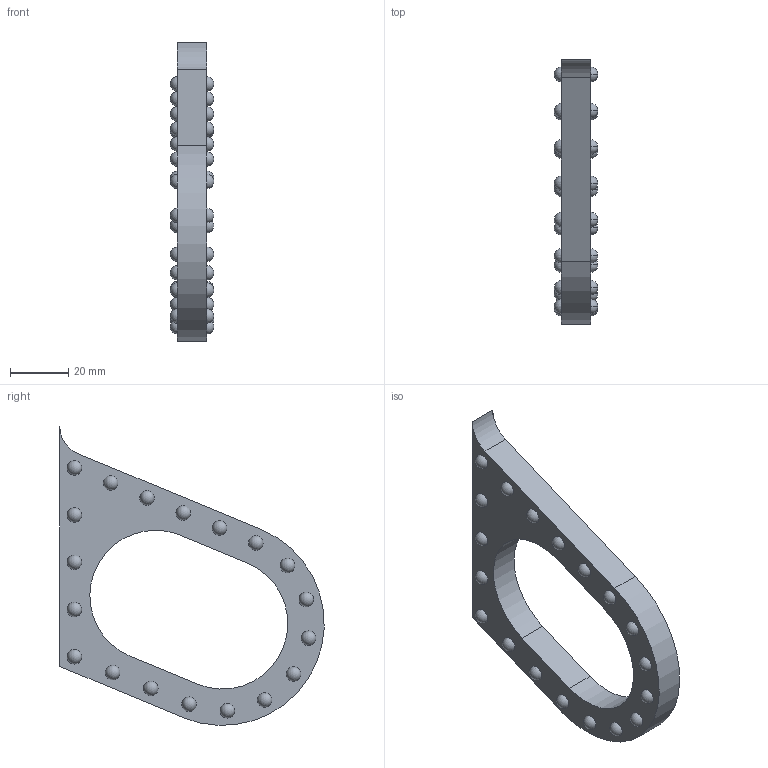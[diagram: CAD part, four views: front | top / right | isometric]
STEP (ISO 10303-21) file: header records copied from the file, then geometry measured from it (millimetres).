
FILE_DESCRIPTION (( 'STEP AP214' ), '1' );
FILE_NAME ('Grip_Middle.step', '2013-11-06T14:31:01', ( 'elpi' ), ( '' ), 'SwSTEP 2.0', 'SolidWorks 2013', '' );
FILE_SCHEMA (( 'AUTOMOTIVE_DESIGN' ));
Length unit declared in the file: millimetre
Products named in the file (1): Grip_Middle
Bounding box: 14.98 x 90.86 x 102.69 mm (x, y, z)
Volume: 35762.4 mm3; surface area: 12748.7 mm2
Topology: 1 solids, 1 shells, 69 faces, 277 edges, 172 vertices
Faces by surface type: sphere 57, plane 7, cylinder 5
Entity records: 1846 total; most frequent: DIRECTION 370, CARTESIAN_POINT 291, ORIENTED_EDGE 250, AXIS2_PLACEMENT_3D 175, EDGE_CURVE 125, EDGE_LOOP 109, CIRCLE 105, VERTEX_POINT 96
